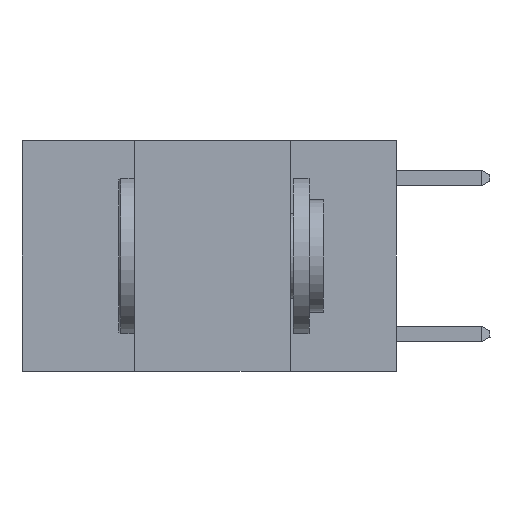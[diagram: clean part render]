
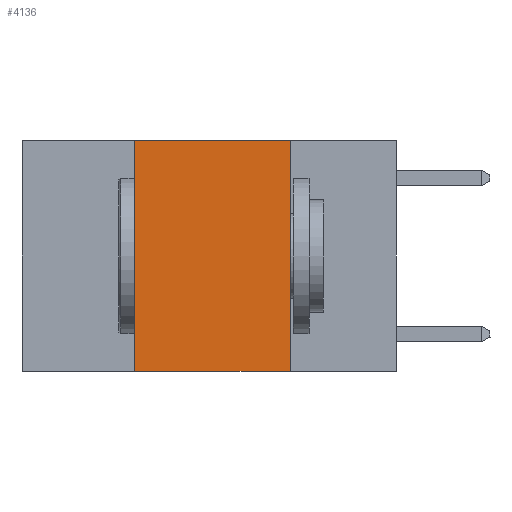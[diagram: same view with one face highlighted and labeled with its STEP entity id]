
A CAD part, left-side view. The second image highlights one B-rep face of the part: STEP entity #4136.
In plain terms, the highlighted planar face has unit normal (-1, 0, 0).
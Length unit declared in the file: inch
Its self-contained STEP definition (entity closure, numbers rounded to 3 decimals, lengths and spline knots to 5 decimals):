
#1051 = CARTESIAN_POINT ( 'NONE',  ( 0., 0.6, 0. ) ) ;
#1104 = LINE ( 'NONE', #17721, #17734 ) ;
#2156 = EDGE_CURVE ( 'NONE', #26150, #9042, #10813, .T. ) ;
#2711 = VECTOR ( 'NONE', #20312, 39.37008 ) ;
#4136 = ADVANCED_FACE ( 'NONE', ( #23998 ), #5301, .F. ) ;
#4355 = CARTESIAN_POINT ( 'NONE',  ( 0., 0.42, -0.37 ) ) ;
#4421 = CARTESIAN_POINT ( 'NONE',  ( 0., 0.17, 0. ) ) ;
#5164 = DIRECTION ( 'NONE',  ( 1., 0., 0. ) ) ;
#5301 = PLANE ( 'NONE',  #19170 ) ;
#5362 = DIRECTION ( 'NONE',  ( 0., 0., 1. ) ) ;
#6989 = EDGE_LOOP ( 'NONE', ( #12176, #12914, #18920, #24985 ) ) ;
#9042 = VERTEX_POINT ( 'NONE', #4421 ) ;
#9738 = LINE ( 'NONE', #16449, #14763 ) ;
#10813 = LINE ( 'NONE', #23589, #17222 ) ;
#11197 = EDGE_CURVE ( 'NONE', #9042, #14577, #20575, .T. ) ;
#11241 = CARTESIAN_POINT ( 'NONE',  ( 0., 0.17, -0.37 ) ) ;
#12176 = ORIENTED_EDGE ( 'NONE', *, *, #11197, .F. ) ;
#12914 = ORIENTED_EDGE ( 'NONE', *, *, #2156, .F. ) ;
#13013 = DIRECTION ( 'NONE',  ( 0., -1., 0. ) ) ;
#13558 = DIRECTION ( 'NONE',  ( 0., 0., -1. ) ) ;
#14223 = EDGE_CURVE ( 'NONE', #18802, #26150, #1104, .T. ) ;
#14577 = VERTEX_POINT ( 'NONE', #11241 ) ;
#14763 = VECTOR ( 'NONE', #18102, 39.37008 ) ;
#16449 = CARTESIAN_POINT ( 'NONE',  ( 0., 0.6, -0.37 ) ) ;
#17222 = VECTOR ( 'NONE', #13013, 39.37008 ) ;
#17721 = CARTESIAN_POINT ( 'NONE',  ( 0., 0.42, 0. ) ) ;
#17734 = VECTOR ( 'NONE', #5362, 39.37008 ) ;
#17824 = CARTESIAN_POINT ( 'NONE',  ( 0., 0.42, 0. ) ) ;
#18102 = DIRECTION ( 'NONE',  ( 0., -1., 0. ) ) ;
#18734 = EDGE_CURVE ( 'NONE', #18802, #14577, #9738, .T. ) ;
#18802 = VERTEX_POINT ( 'NONE', #4355 ) ;
#18920 = ORIENTED_EDGE ( 'NONE', *, *, #14223, .F. ) ;
#19170 = AXIS2_PLACEMENT_3D ( 'NONE', #1051, #5164, #13558 ) ;
#20312 = DIRECTION ( 'NONE',  ( 0., 0., -1. ) ) ;
#20448 = CARTESIAN_POINT ( 'NONE',  ( 0., 0.17, 0. ) ) ;
#20575 = LINE ( 'NONE', #20448, #2711 ) ;
#23589 = CARTESIAN_POINT ( 'NONE',  ( 0., 0.6, 0. ) ) ;
#23998 = FACE_OUTER_BOUND ( 'NONE', #6989, .T. ) ;
#24985 = ORIENTED_EDGE ( 'NONE', *, *, #18734, .T. ) ;
#26150 = VERTEX_POINT ( 'NONE', #17824 ) ;
